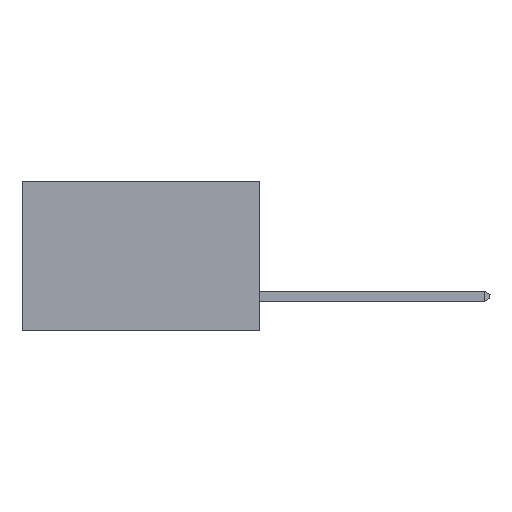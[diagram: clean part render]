
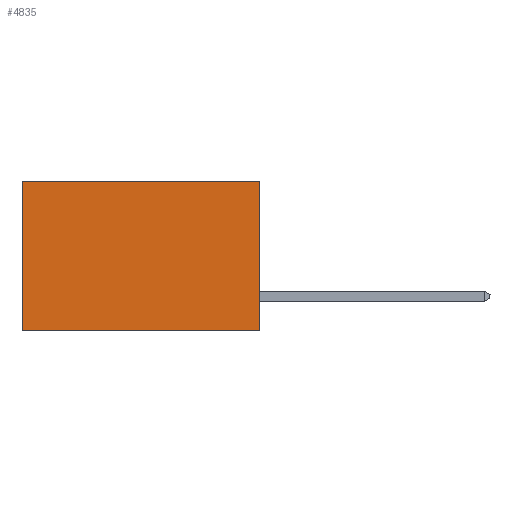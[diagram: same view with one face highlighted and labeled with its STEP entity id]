
A CAD part, left-side view. The second image highlights one B-rep face of the part: STEP entity #4835.
In plain terms, the highlighted planar face has unit normal (-1, 0, 0).
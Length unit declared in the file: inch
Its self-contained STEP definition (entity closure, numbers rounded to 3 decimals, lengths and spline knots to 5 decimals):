
#192 = LINE ( 'NONE', #6915, #5389 ) ;
#929 = ORIENTED_EDGE ( 'NONE', *, *, #6873, .T. ) ;
#1042 = ORIENTED_EDGE ( 'NONE', *, *, #3158, .F. ) ;
#1082 = VECTOR ( 'NONE', #4626, 39.37008 ) ;
#1165 = ORIENTED_EDGE ( 'NONE', *, *, #6909, .F. ) ;
#1263 = ORIENTED_EDGE ( 'NONE', *, *, #3142, .T. ) ;
#1293 = LINE ( 'NONE', #4822, #1082 ) ;
#1802 = VERTEX_POINT ( 'NONE', #2748 ) ;
#1836 = VECTOR ( 'NONE', #6761, 39.37008 ) ;
#2196 = VERTEX_POINT ( 'NONE', #2893 ) ;
#2503 = VERTEX_POINT ( 'NONE', #6098 ) ;
#2616 = VECTOR ( 'NONE', #4288, 39.37008 ) ;
#2748 = CARTESIAN_POINT ( 'NONE',  ( 0.277, 0., -0.37 ) ) ;
#2775 = VERTEX_POINT ( 'NONE', #7518 ) ;
#2893 = CARTESIAN_POINT ( 'NONE',  ( 0.277, 0., 0. ) ) ;
#3142 = EDGE_CURVE ( 'NONE', #2196, #2775, #192, .T. ) ;
#3158 = EDGE_CURVE ( 'NONE', #1802, #2503, #3561, .T. ) ;
#3561 = LINE ( 'NONE', #6808, #1836 ) ;
#4288 = DIRECTION ( 'NONE',  ( 0., 0., -1. ) ) ;
#4370 = LINE ( 'NONE', #4519, #2616 ) ;
#4519 = CARTESIAN_POINT ( 'NONE',  ( 0.277, 0., -0.37 ) ) ;
#4626 = DIRECTION ( 'NONE',  ( 0., 0., -1. ) ) ;
#4822 = CARTESIAN_POINT ( 'NONE',  ( 0.277, 0.59, -0.37 ) ) ;
#4835 = ADVANCED_FACE ( 'NONE', ( #5096 ), #5973, .F. ) ;
#5096 = FACE_OUTER_BOUND ( 'NONE', #5690, .T. ) ;
#5199 = AXIS2_PLACEMENT_3D ( 'NONE', #5271, #5846, #7106 ) ;
#5271 = CARTESIAN_POINT ( 'NONE',  ( 0.277, 0., -0.37 ) ) ;
#5389 = VECTOR ( 'NONE', #6785, 39.37008 ) ;
#5690 = EDGE_LOOP ( 'NONE', ( #929, #1042, #1165, #1263 ) ) ;
#5846 = DIRECTION ( 'NONE',  ( 1., 0., 0. ) ) ;
#5973 = PLANE ( 'NONE',  #5199 ) ;
#6098 = CARTESIAN_POINT ( 'NONE',  ( 0.277, 0.59, -0.37 ) ) ;
#6761 = DIRECTION ( 'NONE',  ( 0., 1., 0. ) ) ;
#6785 = DIRECTION ( 'NONE',  ( 0., 1., 0. ) ) ;
#6808 = CARTESIAN_POINT ( 'NONE',  ( 0.277, 0., -0.37 ) ) ;
#6873 = EDGE_CURVE ( 'NONE', #2775, #2503, #1293, .T. ) ;
#6909 = EDGE_CURVE ( 'NONE', #2196, #1802, #4370, .T. ) ;
#6915 = CARTESIAN_POINT ( 'NONE',  ( 0.277, 0., 0. ) ) ;
#7106 = DIRECTION ( 'NONE',  ( 0., 0., -1. ) ) ;
#7518 = CARTESIAN_POINT ( 'NONE',  ( 0.277, 0.59, 0. ) ) ;
